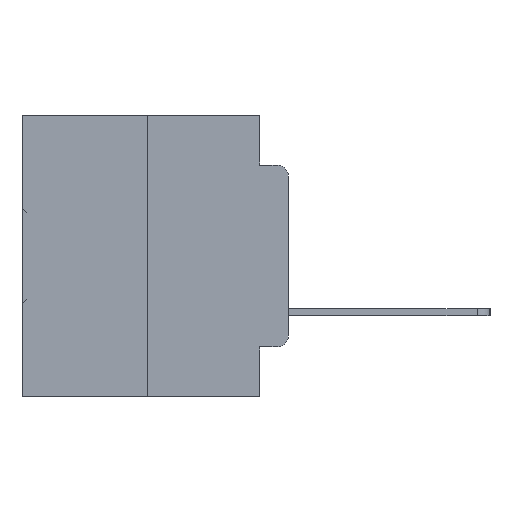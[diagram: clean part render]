
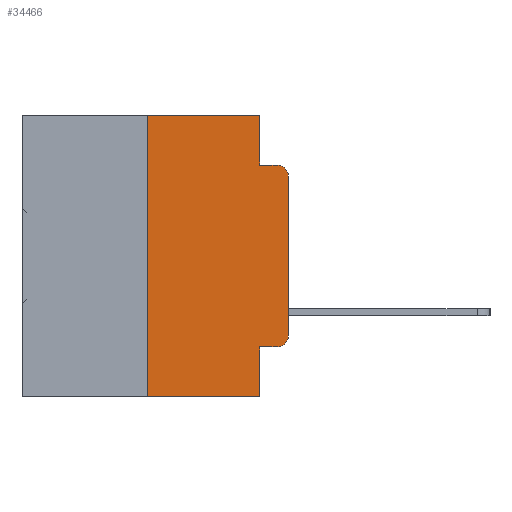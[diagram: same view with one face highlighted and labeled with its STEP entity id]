
A CAD part, left-side view. The second image highlights one B-rep face of the part: STEP entity #34466.
In plain terms, the highlighted planar face has unit normal (-1, 0, 0).
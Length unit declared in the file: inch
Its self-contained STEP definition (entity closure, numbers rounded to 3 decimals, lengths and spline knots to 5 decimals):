
#492 = ORIENTED_EDGE ( 'NONE', *, *, #27060, .T. ) ;
#518 = ORIENTED_EDGE ( 'NONE', *, *, #1147, .T. ) ;
#748 = LINE ( 'NONE', #23225, #28517 ) ;
#1147 = EDGE_CURVE ( 'NONE', #10663, #24694, #28111, .T. ) ;
#1153 = CARTESIAN_POINT ( 'NONE',  ( 0., 0.02, -0.0885 ) ) ;
#1618 = VECTOR ( 'NONE', #21729, 39.37008 ) ;
#1714 = CARTESIAN_POINT ( 'NONE',  ( 0., 0.051, 0. ) ) ;
#2043 = EDGE_CURVE ( 'NONE', #24694, #21926, #7675, .T. ) ;
#2258 = AXIS2_PLACEMENT_3D ( 'NONE', #24061, #30963, #15110 ) ;
#3483 = CARTESIAN_POINT ( 'NONE',  ( 0., 0., -0.1085 ) ) ;
#3932 = EDGE_CURVE ( 'NONE', #21926, #21162, #19204, .T. ) ;
#3970 = LINE ( 'NONE', #11508, #31528 ) ;
#4443 = VERTEX_POINT ( 'NONE', #7299 ) ;
#4921 = VECTOR ( 'NONE', #26058, 39.37008 ) ;
#5294 = VERTEX_POINT ( 'NONE', #31297 ) ;
#7299 = CARTESIAN_POINT ( 'NONE',  ( 0., 0.25, -0.5 ) ) ;
#7675 = LINE ( 'NONE', #10894, #21803 ) ;
#7755 = CARTESIAN_POINT ( 'NONE',  ( 0., 0.02, -0.4115 ) ) ;
#8347 = CARTESIAN_POINT ( 'NONE',  ( 0., 0.051, 0. ) ) ;
#8515 = CARTESIAN_POINT ( 'NONE',  ( 0., 0.051, -0.0885 ) ) ;
#10098 = FACE_OUTER_BOUND ( 'NONE', #30045, .T. ) ;
#10663 = VERTEX_POINT ( 'NONE', #7755 ) ;
#10894 = CARTESIAN_POINT ( 'NONE',  ( 0., 0., 0. ) ) ;
#10924 = DIRECTION ( 'NONE',  ( 0., 0., 1. ) ) ;
#11244 = CARTESIAN_POINT ( 'NONE',  ( 0., 0.473, 0. ) ) ;
#11508 = CARTESIAN_POINT ( 'NONE',  ( 0., 0.25, 0. ) ) ;
#11633 = DIRECTION ( 'NONE',  ( 0., 0., 1. ) ) ;
#12174 = LINE ( 'NONE', #23398, #4921 ) ;
#12238 = CARTESIAN_POINT ( 'NONE',  ( 0., 0.051, -0.4115 ) ) ;
#12342 = VECTOR ( 'NONE', #18892, 39.37008 ) ;
#12544 = VERTEX_POINT ( 'NONE', #31891 ) ;
#12680 = VERTEX_POINT ( 'NONE', #21927 ) ;
#12735 = DIRECTION ( 'NONE',  ( 0., -1., 0. ) ) ;
#13186 = LINE ( 'NONE', #8347, #12342 ) ;
#13729 = VECTOR ( 'NONE', #14878, 39.37008 ) ;
#13906 = DIRECTION ( 'NONE',  ( 1., 0., 0. ) ) ;
#14564 = AXIS2_PLACEMENT_3D ( 'NONE', #11244, #13906, #32366 ) ;
#14633 = EDGE_CURVE ( 'NONE', #19898, #12544, #13186, .T. ) ;
#14878 = DIRECTION ( 'NONE',  ( 0., -1., 0. ) ) ;
#15110 = DIRECTION ( 'NONE',  ( 0., 0., -1. ) ) ;
#15935 = CARTESIAN_POINT ( 'NONE',  ( 0., 0.051, 0. ) ) ;
#16287 = DIRECTION ( 'NONE',  ( -1., 0., 0. ) ) ;
#16324 = CARTESIAN_POINT ( 'NONE',  ( 0., 0.02, -0.3915 ) ) ;
#16394 = EDGE_CURVE ( 'NONE', #4443, #5294, #3970, .T. ) ;
#18346 = EDGE_CURVE ( 'NONE', #12544, #21162, #23084, .T. ) ;
#18892 = DIRECTION ( 'NONE',  ( 0., 0., -1. ) ) ;
#19204 = CIRCLE ( 'NONE', #2258, 0.02 ) ;
#19898 = VERTEX_POINT ( 'NONE', #15935 ) ;
#20303 = ORIENTED_EDGE ( 'NONE', *, *, #2043, .T. ) ;
#21162 = VERTEX_POINT ( 'NONE', #1153 ) ;
#21556 = LINE ( 'NONE', #12238, #13729 ) ;
#21729 = DIRECTION ( 'NONE',  ( 0., -1., 0. ) ) ;
#21803 = VECTOR ( 'NONE', #10924, 39.37008 ) ;
#21926 = VERTEX_POINT ( 'NONE', #3483 ) ;
#21927 = CARTESIAN_POINT ( 'NONE',  ( 0., 0.051, -0.5 ) ) ;
#22504 = VECTOR ( 'NONE', #23245, 39.37008 ) ;
#23084 = LINE ( 'NONE', #8515, #1618 ) ;
#23196 = ORIENTED_EDGE ( 'NONE', *, *, #3932, .T. ) ;
#23225 = CARTESIAN_POINT ( 'NONE',  ( 0., 0.473, 0. ) ) ;
#23245 = DIRECTION ( 'NONE',  ( 0., 0., -1. ) ) ;
#23371 = LINE ( 'NONE', #1714, #22504 ) ;
#23398 = CARTESIAN_POINT ( 'NONE',  ( 0., 0.473, -0.5 ) ) ;
#23614 = ORIENTED_EDGE ( 'NONE', *, *, #18346, .F. ) ;
#24020 = ORIENTED_EDGE ( 'NONE', *, *, #14633, .F. ) ;
#24061 = CARTESIAN_POINT ( 'NONE',  ( 0., 0.02, -0.1085 ) ) ;
#24143 = ORIENTED_EDGE ( 'NONE', *, *, #31492, .F. ) ;
#24596 = ORIENTED_EDGE ( 'NONE', *, *, #16394, .F. ) ;
#24694 = VERTEX_POINT ( 'NONE', #28285 ) ;
#24794 = CARTESIAN_POINT ( 'NONE',  ( 0., 0.051, -0.4115 ) ) ;
#25297 = EDGE_CURVE ( 'NONE', #27672, #12680, #23371, .T. ) ;
#25422 = ORIENTED_EDGE ( 'NONE', *, *, #25887, .T. ) ;
#25887 = EDGE_CURVE ( 'NONE', #4443, #12680, #12174, .T. ) ;
#26058 = DIRECTION ( 'NONE',  ( 0., -1., 0. ) ) ;
#27060 = EDGE_CURVE ( 'NONE', #27672, #10663, #21556, .T. ) ;
#27086 = PLANE ( 'NONE',  #14564 ) ;
#27663 = ORIENTED_EDGE ( 'NONE', *, *, #25297, .F. ) ;
#27672 = VERTEX_POINT ( 'NONE', #24794 ) ;
#28111 = CIRCLE ( 'NONE', #28747, 0.02 ) ;
#28285 = CARTESIAN_POINT ( 'NONE',  ( 0., 0., -0.3915 ) ) ;
#28517 = VECTOR ( 'NONE', #12735, 39.37008 ) ;
#28747 = AXIS2_PLACEMENT_3D ( 'NONE', #16324, #16287, #29431 ) ;
#29431 = DIRECTION ( 'NONE',  ( 0., 0., -1. ) ) ;
#30045 = EDGE_LOOP ( 'NONE', ( #20303, #23196, #23614, #24020, #24143, #24596, #25422, #27663, #492, #518 ) ) ;
#30963 = DIRECTION ( 'NONE',  ( -1., 0., 0. ) ) ;
#31297 = CARTESIAN_POINT ( 'NONE',  ( 0., 0.25, 0. ) ) ;
#31492 = EDGE_CURVE ( 'NONE', #5294, #19898, #748, .T. ) ;
#31528 = VECTOR ( 'NONE', #11633, 39.37008 ) ;
#31891 = CARTESIAN_POINT ( 'NONE',  ( 0., 0.051, -0.0885 ) ) ;
#32366 = DIRECTION ( 'NONE',  ( 0., 0., -1. ) ) ;
#34466 = ADVANCED_FACE ( 'NONE', ( #10098 ), #27086, .F. ) ;
